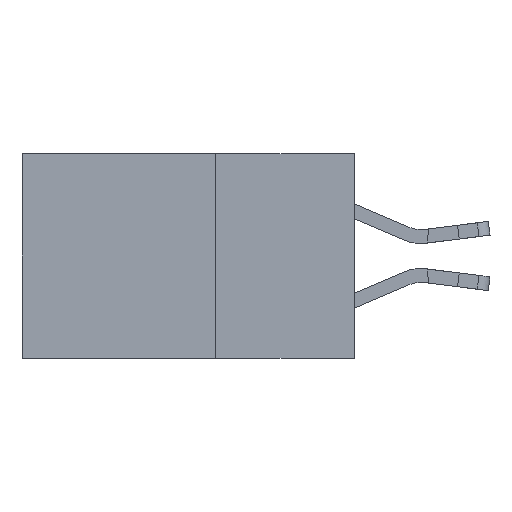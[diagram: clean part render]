
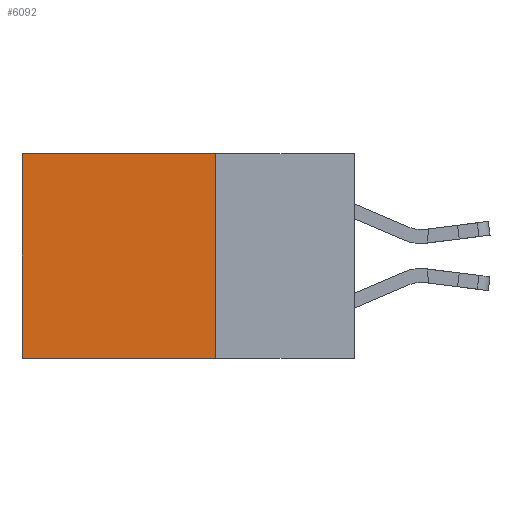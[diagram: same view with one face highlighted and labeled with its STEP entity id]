
A CAD part, left-side view. The second image highlights one B-rep face of the part: STEP entity #6092.
In plain terms, the highlighted planar face has unit normal (-1, 0, 0).
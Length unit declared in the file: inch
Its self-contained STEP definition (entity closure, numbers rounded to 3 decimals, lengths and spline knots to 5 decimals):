
#848 = ORIENTED_EDGE ( 'NONE', *, *, #4414, .F. ) ;
#1052 = VERTEX_POINT ( 'NONE', #5114 ) ;
#1319 = VECTOR ( 'NONE', #13042, 39.37008 ) ;
#1530 = EDGE_LOOP ( 'NONE', ( #2812, #848, #3545, #13169 ) ) ;
#2070 = VERTEX_POINT ( 'NONE', #5837 ) ;
#2179 = CARTESIAN_POINT ( 'NONE',  ( 0.298, 0.25, 0. ) ) ;
#2512 = VERTEX_POINT ( 'NONE', #10138 ) ;
#2648 = DIRECTION ( 'NONE',  ( 0., 0., -1. ) ) ;
#2812 = ORIENTED_EDGE ( 'NONE', *, *, #11523, .T. ) ;
#3265 = VECTOR ( 'NONE', #2648, 39.37008 ) ;
#3545 = ORIENTED_EDGE ( 'NONE', *, *, #8868, .F. ) ;
#3640 = CARTESIAN_POINT ( 'NONE',  ( 0.298, 0.6, 0. ) ) ;
#4269 = FACE_OUTER_BOUND ( 'NONE', #1530, .T. ) ;
#4276 = DIRECTION ( 'NONE',  ( 1., 0., 0. ) ) ;
#4414 = EDGE_CURVE ( 'NONE', #2070, #1052, #6390, .T. ) ;
#4437 = LINE ( 'NONE', #3640, #1319 ) ;
#4632 = VECTOR ( 'NONE', #10699, 39.37008 ) ;
#5114 = CARTESIAN_POINT ( 'NONE',  ( 0.298, 0.6, -0.37 ) ) ;
#5343 = AXIS2_PLACEMENT_3D ( 'NONE', #8016, #4276, #6691 ) ;
#5388 = VERTEX_POINT ( 'NONE', #5630 ) ;
#5630 = CARTESIAN_POINT ( 'NONE',  ( 0.298, 0.25, 0. ) ) ;
#5837 = CARTESIAN_POINT ( 'NONE',  ( 0.298, 0.25, -0.37 ) ) ;
#6092 = ADVANCED_FACE ( 'NONE', ( #4269 ), #10530, .F. ) ;
#6390 = LINE ( 'NONE', #12839, #14044 ) ;
#6442 = LINE ( 'NONE', #8468, #3265 ) ;
#6691 = DIRECTION ( 'NONE',  ( 0., 0., -1. ) ) ;
#8016 = CARTESIAN_POINT ( 'NONE',  ( 0.298, 0.25, 0. ) ) ;
#8468 = CARTESIAN_POINT ( 'NONE',  ( 0.298, 0.25, 0. ) ) ;
#8868 = EDGE_CURVE ( 'NONE', #5388, #2070, #6442, .T. ) ;
#10138 = CARTESIAN_POINT ( 'NONE',  ( 0.298, 0.6, 0. ) ) ;
#10530 = PLANE ( 'NONE',  #5343 ) ;
#10699 = DIRECTION ( 'NONE',  ( 0., 1., 0. ) ) ;
#10896 = EDGE_CURVE ( 'NONE', #5388, #2512, #14172, .T. ) ;
#11523 = EDGE_CURVE ( 'NONE', #2512, #1052, #4437, .T. ) ;
#12839 = CARTESIAN_POINT ( 'NONE',  ( 0.298, 0.25, -0.37 ) ) ;
#13042 = DIRECTION ( 'NONE',  ( 0., 0., -1. ) ) ;
#13169 = ORIENTED_EDGE ( 'NONE', *, *, #10896, .T. ) ;
#14044 = VECTOR ( 'NONE', #15332, 39.37008 ) ;
#14172 = LINE ( 'NONE', #2179, #4632 ) ;
#15332 = DIRECTION ( 'NONE',  ( 0., 1., 0. ) ) ;
